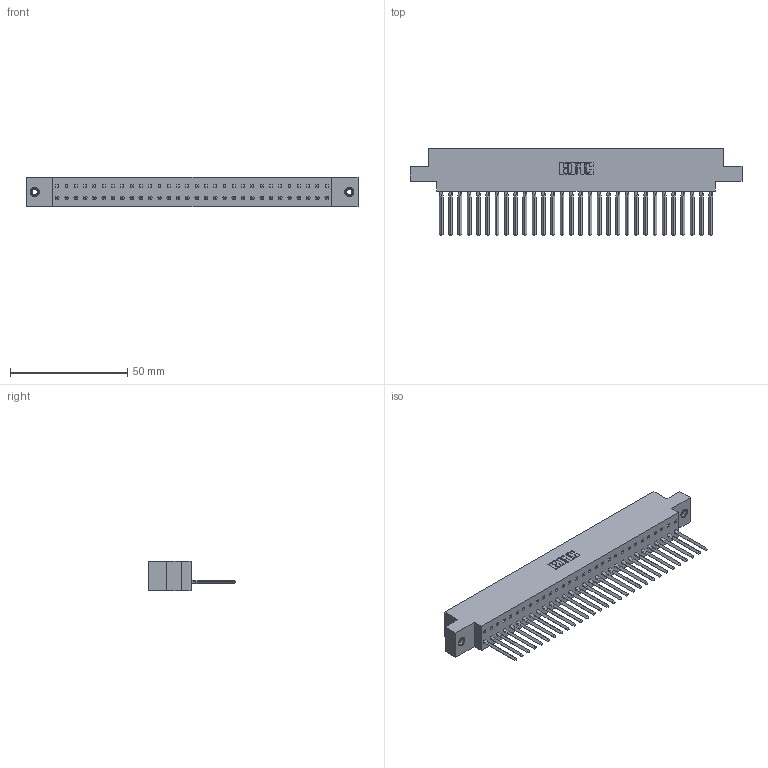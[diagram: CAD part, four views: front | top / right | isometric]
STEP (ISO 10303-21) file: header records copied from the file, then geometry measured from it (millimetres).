
FILE_DESCRIPTION (( 'STEP AP203' ), '1' );
FILE_NAME ('317-030-541-678.STEP', '2020-02-27T20:17:11', ( '' ), ( '' ), 'SwSTEP 2.0', 'SolidWorks 2016', '' );
FILE_SCHEMA (( 'CONFIG_CONTROL_DESIGN' ));
Length unit declared in the file: inch
Products named in the file (4): 317 Part_.156 Dia - TI; 345-250-001_345-250-003-102; 317-030-541-678; 317-290-002_541
Assembly tree (33 placements, depth 2):
  317-030-541-678
    317 Part_.156 Dia - TI
    317-290-002_541  x30
    345-250-001_345-250-003-102  x2
Bounding box: 141.58 x 37.34 x 12.7 mm (x, y, z)
Volume: 22584 mm3; surface area: 31534.1 mm2
Topology: 33 solids, 33 shells, 4722 faces, 13431 edges, 8726 vertices
Faces by surface type: plane 3810, cylinder 776, bspline 120, cone 12, torus 4
Entity records: 46813 total; most frequent: CARTESIAN_POINT 8926, ORIENTED_EDGE 8202, DIRECTION 6771, EDGE_CURVE 4101, LINE 3717, VECTOR 3717, VERTEX_POINT 2722, AXIS2_PLACEMENT_3D 1527
